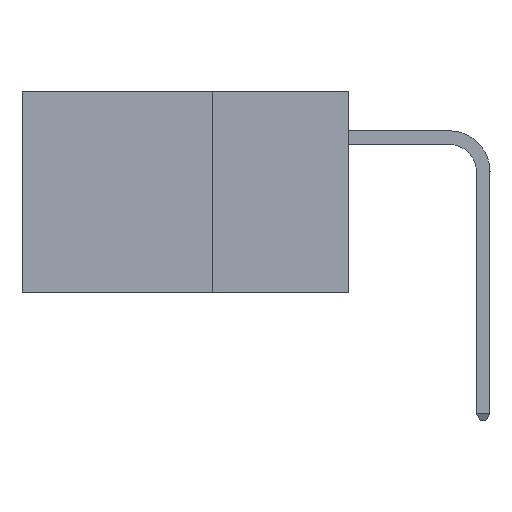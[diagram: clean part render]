
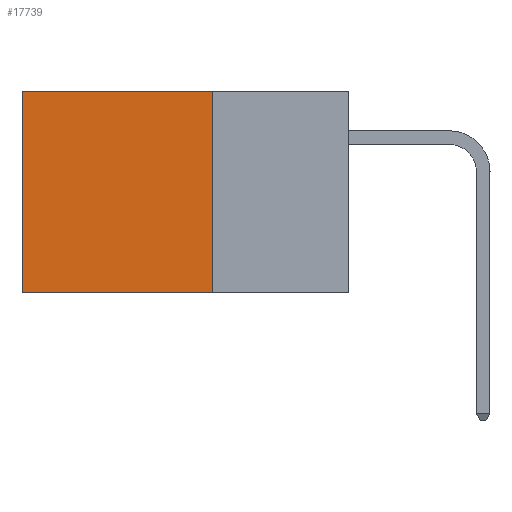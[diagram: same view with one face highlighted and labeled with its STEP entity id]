
A CAD part, left-side view. The second image highlights one B-rep face of the part: STEP entity #17739.
In plain terms, the highlighted planar face has unit normal (-1, 0, 0).
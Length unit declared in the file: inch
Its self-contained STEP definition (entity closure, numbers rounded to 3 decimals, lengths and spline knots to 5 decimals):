
#1555 = DIRECTION ( 'NONE',  ( 0., 0., -1. ) ) ;
#1568 = ORIENTED_EDGE ( 'NONE', *, *, #35817, .F. ) ;
#1974 = VECTOR ( 'NONE', #1555, 39.37008 ) ;
#2278 = DIRECTION ( 'NONE',  ( 1., 0., 0. ) ) ;
#3639 = VERTEX_POINT ( 'NONE', #19823 ) ;
#5976 = CARTESIAN_POINT ( 'NONE',  ( 0.2875, 0.25, 0. ) ) ;
#7136 = DIRECTION ( 'NONE',  ( 0., 1., 0. ) ) ;
#9490 = ORIENTED_EDGE ( 'NONE', *, *, #31200, .F. ) ;
#9859 = AXIS2_PLACEMENT_3D ( 'NONE', #19782, #2278, #22705 ) ;
#10832 = FACE_OUTER_BOUND ( 'NONE', #34043, .T. ) ;
#13019 = ORIENTED_EDGE ( 'NONE', *, *, #34029, .T. ) ;
#13948 = VERTEX_POINT ( 'NONE', #14573 ) ;
#14324 = VECTOR ( 'NONE', #17885, 39.37008 ) ;
#14573 = CARTESIAN_POINT ( 'NONE',  ( 0.2875, 0.25, 0. ) ) ;
#14934 = CARTESIAN_POINT ( 'NONE',  ( 0.2875, 0.25, -0.37 ) ) ;
#17673 = VERTEX_POINT ( 'NONE', #19545 ) ;
#17739 = ADVANCED_FACE ( 'NONE', ( #10832 ), #25445, .F. ) ;
#17885 = DIRECTION ( 'NONE',  ( 0., 1., 0. ) ) ;
#19545 = CARTESIAN_POINT ( 'NONE',  ( 0.2875, 0.6, -0.37 ) ) ;
#19782 = CARTESIAN_POINT ( 'NONE',  ( 0.2875, 0.25, 0. ) ) ;
#19823 = CARTESIAN_POINT ( 'NONE',  ( 0.2875, 0.6, 0. ) ) ;
#20505 = DIRECTION ( 'NONE',  ( 0., 0., -1. ) ) ;
#22660 = VECTOR ( 'NONE', #20505, 39.37008 ) ;
#22705 = DIRECTION ( 'NONE',  ( 0., 0., -1. ) ) ;
#24102 = ORIENTED_EDGE ( 'NONE', *, *, #26652, .T. ) ;
#25033 = VERTEX_POINT ( 'NONE', #28312 ) ;
#25224 = LINE ( 'NONE', #27711, #1974 ) ;
#25445 = PLANE ( 'NONE',  #9859 ) ;
#26652 = EDGE_CURVE ( 'NONE', #3639, #17673, #25224, .T. ) ;
#27375 = CARTESIAN_POINT ( 'NONE',  ( 0.2875, 0.25, 0. ) ) ;
#27681 = LINE ( 'NONE', #27375, #33438 ) ;
#27711 = CARTESIAN_POINT ( 'NONE',  ( 0.2875, 0.6, 0. ) ) ;
#28312 = CARTESIAN_POINT ( 'NONE',  ( 0.2875, 0.25, -0.37 ) ) ;
#29628 = LINE ( 'NONE', #14934, #14324 ) ;
#30221 = LINE ( 'NONE', #5976, #22660 ) ;
#31200 = EDGE_CURVE ( 'NONE', #25033, #17673, #29628, .T. ) ;
#33438 = VECTOR ( 'NONE', #7136, 39.37008 ) ;
#34029 = EDGE_CURVE ( 'NONE', #13948, #3639, #27681, .T. ) ;
#34043 = EDGE_LOOP ( 'NONE', ( #24102, #9490, #1568, #13019 ) ) ;
#35817 = EDGE_CURVE ( 'NONE', #13948, #25033, #30221, .T. ) ;
